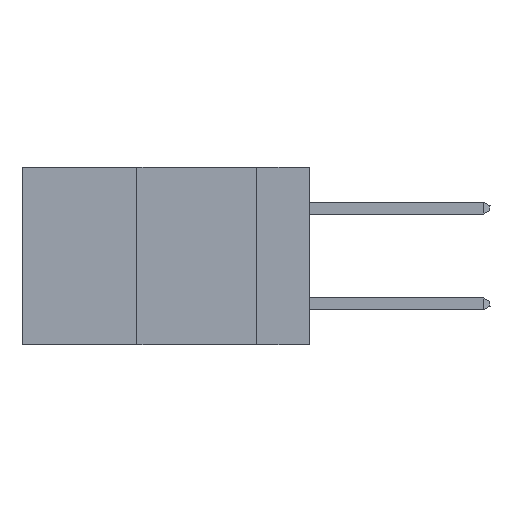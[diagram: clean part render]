
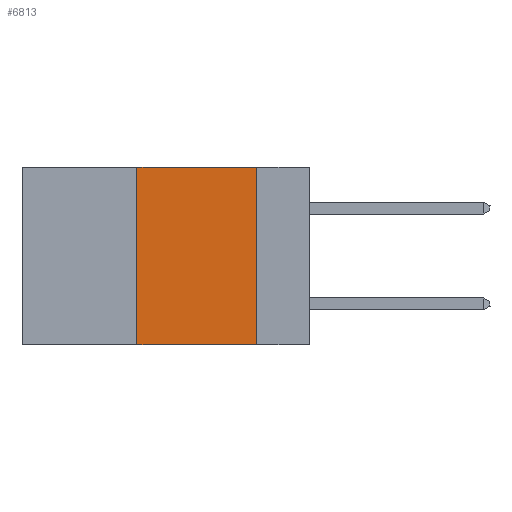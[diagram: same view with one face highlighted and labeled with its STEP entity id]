
A CAD part, left-side view. The second image highlights one B-rep face of the part: STEP entity #6813.
In plain terms, the highlighted planar face has unit normal (-1, 0, 0).
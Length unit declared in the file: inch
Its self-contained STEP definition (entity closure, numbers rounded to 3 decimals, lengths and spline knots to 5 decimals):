
#411 = CARTESIAN_POINT ( 'NONE',  ( 0., 0.11, -0.37 ) ) ;
#586 = CARTESIAN_POINT ( 'NONE',  ( 0., 0.36, 0. ) ) ;
#591 = EDGE_CURVE ( 'NONE', #11965, #1226, #1952, .T. ) ;
#688 = EDGE_CURVE ( 'NONE', #2879, #6273, #12141, .T. ) ;
#1068 = EDGE_LOOP ( 'NONE', ( #1981, #9121, #6587, #5860 ) ) ;
#1111 = DIRECTION ( 'NONE',  ( 0., -1., 0. ) ) ;
#1226 = VERTEX_POINT ( 'NONE', #411 ) ;
#1902 = CARTESIAN_POINT ( 'NONE',  ( 0., 0.36, 0. ) ) ;
#1952 = LINE ( 'NONE', #2638, #6898 ) ;
#1981 = ORIENTED_EDGE ( 'NONE', *, *, #7528, .F. ) ;
#2638 = CARTESIAN_POINT ( 'NONE',  ( 0., 0.6, -0.37 ) ) ;
#2879 = VERTEX_POINT ( 'NONE', #1902 ) ;
#3650 = VECTOR ( 'NONE', #12222, 39.37008 ) ;
#4147 = CARTESIAN_POINT ( 'NONE',  ( 0., 0.6, 0. ) ) ;
#4247 = CARTESIAN_POINT ( 'NONE',  ( 0., 0.6, 0. ) ) ;
#5067 = DIRECTION ( 'NONE',  ( 1., 0., 0. ) ) ;
#5860 = ORIENTED_EDGE ( 'NONE', *, *, #591, .T. ) ;
#5898 = VECTOR ( 'NONE', #1111, 39.37008 ) ;
#6022 = DIRECTION ( 'NONE',  ( 0., 0., 1. ) ) ;
#6204 = PLANE ( 'NONE',  #12458 ) ;
#6258 = VECTOR ( 'NONE', #6022, 39.37008 ) ;
#6273 = VERTEX_POINT ( 'NONE', #11008 ) ;
#6587 = ORIENTED_EDGE ( 'NONE', *, *, #8804, .F. ) ;
#6813 = ADVANCED_FACE ( 'NONE', ( #10918 ), #6204, .F. ) ;
#6898 = VECTOR ( 'NONE', #12096, 39.37008 ) ;
#6934 = LINE ( 'NONE', #586, #6258 ) ;
#6974 = CARTESIAN_POINT ( 'NONE',  ( 0., 0.36, -0.37 ) ) ;
#7528 = EDGE_CURVE ( 'NONE', #6273, #1226, #11863, .T. ) ;
#8804 = EDGE_CURVE ( 'NONE', #11965, #2879, #6934, .T. ) ;
#9121 = ORIENTED_EDGE ( 'NONE', *, *, #688, .F. ) ;
#10918 = FACE_OUTER_BOUND ( 'NONE', #1068, .T. ) ;
#11008 = CARTESIAN_POINT ( 'NONE',  ( 0., 0.11, 0. ) ) ;
#11863 = LINE ( 'NONE', #13386, #3650 ) ;
#11965 = VERTEX_POINT ( 'NONE', #6974 ) ;
#12096 = DIRECTION ( 'NONE',  ( 0., -1., 0. ) ) ;
#12141 = LINE ( 'NONE', #4247, #5898 ) ;
#12222 = DIRECTION ( 'NONE',  ( 0., 0., -1. ) ) ;
#12458 = AXIS2_PLACEMENT_3D ( 'NONE', #4147, #5067, #13533 ) ;
#13386 = CARTESIAN_POINT ( 'NONE',  ( 0., 0.11, 0. ) ) ;
#13533 = DIRECTION ( 'NONE',  ( 0., 0., -1. ) ) ;
